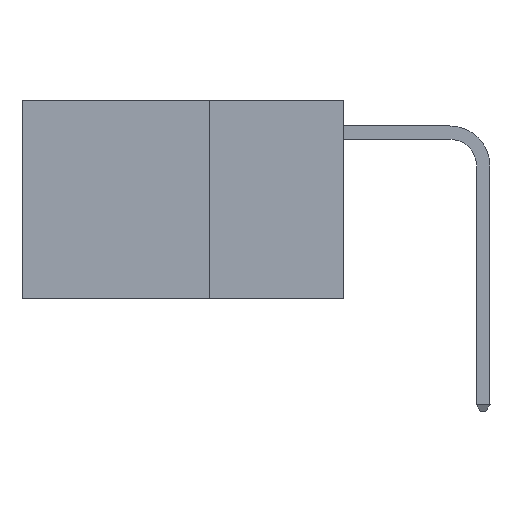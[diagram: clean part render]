
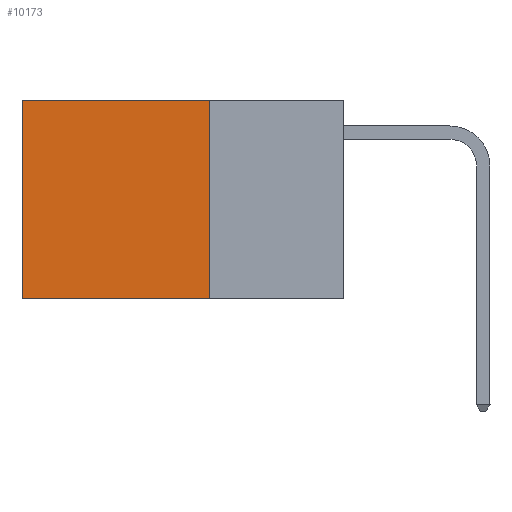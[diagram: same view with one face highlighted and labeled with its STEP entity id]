
A CAD part, left-side view. The second image highlights one B-rep face of the part: STEP entity #10173.
In plain terms, the highlighted planar face has unit normal (-1, 0, 0).
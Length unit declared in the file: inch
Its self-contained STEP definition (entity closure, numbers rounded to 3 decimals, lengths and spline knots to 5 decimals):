
#44 = ORIENTED_EDGE ( 'NONE', *, *, #3187, .T. ) ;
#453 = CARTESIAN_POINT ( 'NONE',  ( 0.2625, 0.25, 0. ) ) ;
#532 = DIRECTION ( 'NONE',  ( 0., 0., -1. ) ) ;
#1139 = LINE ( 'NONE', #453, #3336 ) ;
#1213 = DIRECTION ( 'NONE',  ( 0., 1., 0. ) ) ;
#1336 = DIRECTION ( 'NONE',  ( 0., 0., -1. ) ) ;
#1748 = EDGE_LOOP ( 'NONE', ( #10680, #7712, #5773, #44 ) ) ;
#2397 = EDGE_CURVE ( 'NONE', #10049, #2841, #1139, .T. ) ;
#2771 = VERTEX_POINT ( 'NONE', #11045 ) ;
#2841 = VERTEX_POINT ( 'NONE', #10263 ) ;
#2901 = LINE ( 'NONE', #6300, #7448 ) ;
#3069 = CARTESIAN_POINT ( 'NONE',  ( 0.2625, 0.25, 0. ) ) ;
#3187 = EDGE_CURVE ( 'NONE', #10049, #2771, #7983, .T. ) ;
#3336 = VECTOR ( 'NONE', #1336, 39.37008 ) ;
#5125 = PLANE ( 'NONE',  #11227 ) ;
#5622 = VECTOR ( 'NONE', #1213, 39.37008 ) ;
#5773 = ORIENTED_EDGE ( 'NONE', *, *, #2397, .F. ) ;
#5822 = CARTESIAN_POINT ( 'NONE',  ( 0.2625, 0.25, -0.37 ) ) ;
#6029 = DIRECTION ( 'NONE',  ( 1., 0., 0. ) ) ;
#6300 = CARTESIAN_POINT ( 'NONE',  ( 0.2625, 0.6, 0. ) ) ;
#6757 = EDGE_CURVE ( 'NONE', #2841, #9211, #8319, .T. ) ;
#6912 = CARTESIAN_POINT ( 'NONE',  ( 0.2625, 0.25, 0. ) ) ;
#7448 = VECTOR ( 'NONE', #10751, 39.37008 ) ;
#7712 = ORIENTED_EDGE ( 'NONE', *, *, #6757, .F. ) ;
#7983 = LINE ( 'NONE', #10671, #10097 ) ;
#8156 = EDGE_CURVE ( 'NONE', #2771, #9211, #2901, .T. ) ;
#8319 = LINE ( 'NONE', #5822, #5622 ) ;
#9211 = VERTEX_POINT ( 'NONE', #9692 ) ;
#9692 = CARTESIAN_POINT ( 'NONE',  ( 0.2625, 0.6, -0.37 ) ) ;
#10049 = VERTEX_POINT ( 'NONE', #3069 ) ;
#10097 = VECTOR ( 'NONE', #11620, 39.37008 ) ;
#10173 = ADVANCED_FACE ( 'NONE', ( #11575 ), #5125, .F. ) ;
#10263 = CARTESIAN_POINT ( 'NONE',  ( 0.2625, 0.25, -0.37 ) ) ;
#10671 = CARTESIAN_POINT ( 'NONE',  ( 0.2625, 0.25, 0. ) ) ;
#10680 = ORIENTED_EDGE ( 'NONE', *, *, #8156, .T. ) ;
#10751 = DIRECTION ( 'NONE',  ( 0., 0., -1. ) ) ;
#11045 = CARTESIAN_POINT ( 'NONE',  ( 0.2625, 0.6, 0. ) ) ;
#11227 = AXIS2_PLACEMENT_3D ( 'NONE', #6912, #6029, #532 ) ;
#11575 = FACE_OUTER_BOUND ( 'NONE', #1748, .T. ) ;
#11620 = DIRECTION ( 'NONE',  ( 0., 1., 0. ) ) ;
